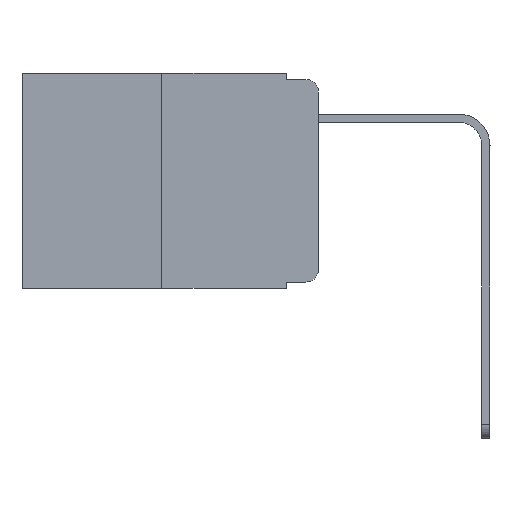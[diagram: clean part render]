
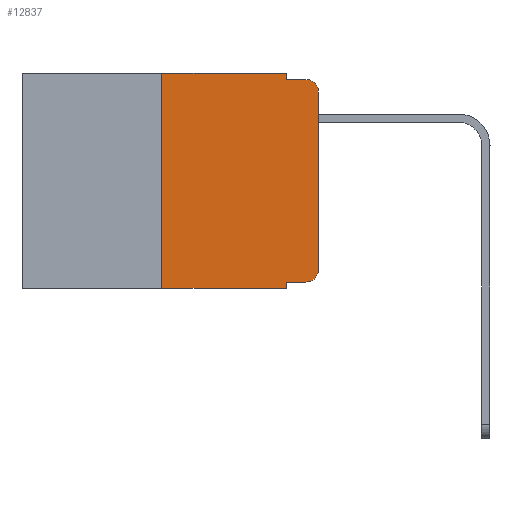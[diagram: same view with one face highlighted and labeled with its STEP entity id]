
A CAD part, left-side view. The second image highlights one B-rep face of the part: STEP entity #12837.
In plain terms, the highlighted planar face has unit normal (-1, 0, 0).
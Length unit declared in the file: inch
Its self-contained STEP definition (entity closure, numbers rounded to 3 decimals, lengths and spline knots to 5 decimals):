
#89 = ORIENTED_EDGE ( 'NONE', *, *, #12052, .F. ) ;
#463 = VECTOR ( 'NONE', #507, 39.37008 ) ;
#507 = DIRECTION ( 'NONE',  ( 0., -1., 0. ) ) ;
#642 = CARTESIAN_POINT ( 'NONE',  ( 0., 0.25, -0.343 ) ) ;
#749 = EDGE_CURVE ( 'NONE', #4454, #2607, #9266, .T. ) ;
#800 = VERTEX_POINT ( 'NONE', #1418 ) ;
#810 = DIRECTION ( 'NONE',  ( -1., 0., 0. ) ) ;
#879 = DIRECTION ( 'NONE',  ( 0., 0., -1. ) ) ;
#885 = CIRCLE ( 'NONE', #10780, 0.02 ) ;
#1011 = VECTOR ( 'NONE', #6478, 39.37008 ) ;
#1111 = EDGE_CURVE ( 'NONE', #8377, #2607, #11007, .T. ) ;
#1223 = VECTOR ( 'NONE', #8650, 39.37008 ) ;
#1232 = VECTOR ( 'NONE', #5985, 39.37008 ) ;
#1362 = CARTESIAN_POINT ( 'NONE',  ( 0., 0.051, -0.333 ) ) ;
#1374 = VECTOR ( 'NONE', #6112, 39.37008 ) ;
#1418 = CARTESIAN_POINT ( 'NONE',  ( 0., 0., -0.03 ) ) ;
#1816 = DIRECTION ( 'NONE',  ( 0., -1., 0. ) ) ;
#2028 = LINE ( 'NONE', #12562, #463 ) ;
#2278 = CARTESIAN_POINT ( 'NONE',  ( 0., 0., 0. ) ) ;
#2340 = DIRECTION ( 'NONE',  ( 0., 0., -1. ) ) ;
#2548 = CARTESIAN_POINT ( 'NONE',  ( 0., 0.051, -0.01 ) ) ;
#2550 = EDGE_CURVE ( 'NONE', #4454, #6482, #9508, .T. ) ;
#2607 = VERTEX_POINT ( 'NONE', #5869 ) ;
#2856 = VERTEX_POINT ( 'NONE', #3815 ) ;
#2864 = LINE ( 'NONE', #2278, #5373 ) ;
#2952 = AXIS2_PLACEMENT_3D ( 'NONE', #12928, #6919, #879 ) ;
#3260 = CARTESIAN_POINT ( 'NONE',  ( 0., 0.051, 0. ) ) ;
#3293 = ORIENTED_EDGE ( 'NONE', *, *, #11639, .T. ) ;
#3378 = ORIENTED_EDGE ( 'NONE', *, *, #3754, .T. ) ;
#3754 = EDGE_CURVE ( 'NONE', #10993, #800, #2864, .T. ) ;
#3815 = CARTESIAN_POINT ( 'NONE',  ( 0., 0.02, -0.333 ) ) ;
#3816 = ORIENTED_EDGE ( 'NONE', *, *, #749, .T. ) ;
#4032 = PLANE ( 'NONE',  #2952 ) ;
#4085 = CARTESIAN_POINT ( 'NONE',  ( 0., 0., -0.313 ) ) ;
#4176 = CIRCLE ( 'NONE', #12041, 0.02 ) ;
#4454 = VERTEX_POINT ( 'NONE', #642 ) ;
#4610 = ORIENTED_EDGE ( 'NONE', *, *, #2550, .F. ) ;
#4906 = LINE ( 'NONE', #11901, #1232 ) ;
#5373 = VECTOR ( 'NONE', #5375, 39.37008 ) ;
#5375 = DIRECTION ( 'NONE',  ( 0., 0., 1. ) ) ;
#5533 = ORIENTED_EDGE ( 'NONE', *, *, #11355, .T. ) ;
#5835 = ORIENTED_EDGE ( 'NONE', *, *, #8051, .T. ) ;
#5849 = CARTESIAN_POINT ( 'NONE',  ( 0., 0.051, -0.333 ) ) ;
#5869 = CARTESIAN_POINT ( 'NONE',  ( 0., 0.051, -0.343 ) ) ;
#5890 = DIRECTION ( 'NONE',  ( 0., 0., -1. ) ) ;
#5919 = LINE ( 'NONE', #2548, #1011 ) ;
#5985 = DIRECTION ( 'NONE',  ( 0., 0., -1. ) ) ;
#6112 = DIRECTION ( 'NONE',  ( 0., 0., -1. ) ) ;
#6478 = DIRECTION ( 'NONE',  ( 0., -1., 0. ) ) ;
#6482 = VERTEX_POINT ( 'NONE', #9096 ) ;
#6560 = CARTESIAN_POINT ( 'NONE',  ( 0., 0.051, -0.01 ) ) ;
#6687 = ORIENTED_EDGE ( 'NONE', *, *, #8035, .F. ) ;
#6694 = CARTESIAN_POINT ( 'NONE',  ( 0., 0.25, 0. ) ) ;
#6919 = DIRECTION ( 'NONE',  ( 1., 0., 0. ) ) ;
#7156 = EDGE_LOOP ( 'NONE', ( #3378, #5533, #89, #6687, #12386, #4610, #3816, #12101, #5835, #3293 ) ) ;
#7795 = EDGE_CURVE ( 'NONE', #6482, #11853, #2028, .T. ) ;
#7906 = CARTESIAN_POINT ( 'NONE',  ( 0., 0.02, -0.313 ) ) ;
#8035 = EDGE_CURVE ( 'NONE', #11853, #10657, #4906, .T. ) ;
#8051 = EDGE_CURVE ( 'NONE', #8377, #2856, #12910, .T. ) ;
#8052 = VERTEX_POINT ( 'NONE', #8863 ) ;
#8377 = VERTEX_POINT ( 'NONE', #1362 ) ;
#8650 = DIRECTION ( 'NONE',  ( 0., -1., 0. ) ) ;
#8863 = CARTESIAN_POINT ( 'NONE',  ( 0., 0.02, -0.01 ) ) ;
#9096 = CARTESIAN_POINT ( 'NONE',  ( 0., 0.25, 0. ) ) ;
#9266 = LINE ( 'NONE', #9588, #1223 ) ;
#9508 = LINE ( 'NONE', #6694, #12023 ) ;
#9588 = CARTESIAN_POINT ( 'NONE',  ( 0., 0.473, -0.343 ) ) ;
#9789 = DIRECTION ( 'NONE',  ( 0., 0., 1. ) ) ;
#10110 = CARTESIAN_POINT ( 'NONE',  ( 0., 0.051, 0. ) ) ;
#10505 = DIRECTION ( 'NONE',  ( -1., 0., 0. ) ) ;
#10657 = VERTEX_POINT ( 'NONE', #6560 ) ;
#10780 = AXIS2_PLACEMENT_3D ( 'NONE', #12502, #10505, #2340 ) ;
#10993 = VERTEX_POINT ( 'NONE', #4085 ) ;
#11007 = LINE ( 'NONE', #3260, #1374 ) ;
#11355 = EDGE_CURVE ( 'NONE', #800, #8052, #885, .T. ) ;
#11633 = VECTOR ( 'NONE', #1816, 39.37008 ) ;
#11639 = EDGE_CURVE ( 'NONE', #2856, #10993, #4176, .T. ) ;
#11853 = VERTEX_POINT ( 'NONE', #10110 ) ;
#11901 = CARTESIAN_POINT ( 'NONE',  ( 0., 0.051, 0. ) ) ;
#12023 = VECTOR ( 'NONE', #9789, 39.37008 ) ;
#12041 = AXIS2_PLACEMENT_3D ( 'NONE', #7906, #810, #5890 ) ;
#12052 = EDGE_CURVE ( 'NONE', #10657, #8052, #5919, .T. ) ;
#12101 = ORIENTED_EDGE ( 'NONE', *, *, #1111, .F. ) ;
#12324 = FACE_OUTER_BOUND ( 'NONE', #7156, .T. ) ;
#12386 = ORIENTED_EDGE ( 'NONE', *, *, #7795, .F. ) ;
#12502 = CARTESIAN_POINT ( 'NONE',  ( 0., 0.02, -0.03 ) ) ;
#12562 = CARTESIAN_POINT ( 'NONE',  ( 0., 0.473, 0. ) ) ;
#12837 = ADVANCED_FACE ( 'NONE', ( #12324 ), #4032, .F. ) ;
#12910 = LINE ( 'NONE', #5849, #11633 ) ;
#12928 = CARTESIAN_POINT ( 'NONE',  ( 0., 0.473, 0. ) ) ;
